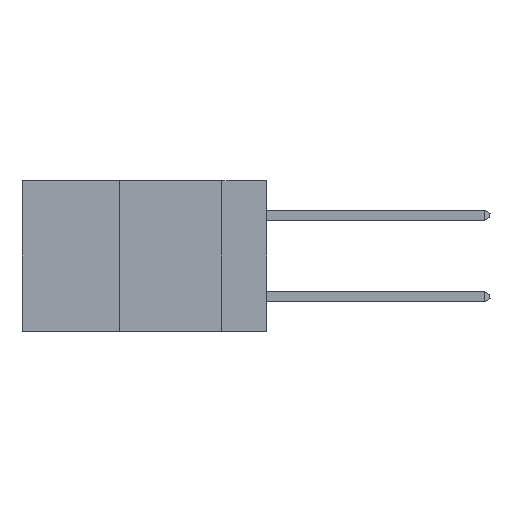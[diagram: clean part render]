
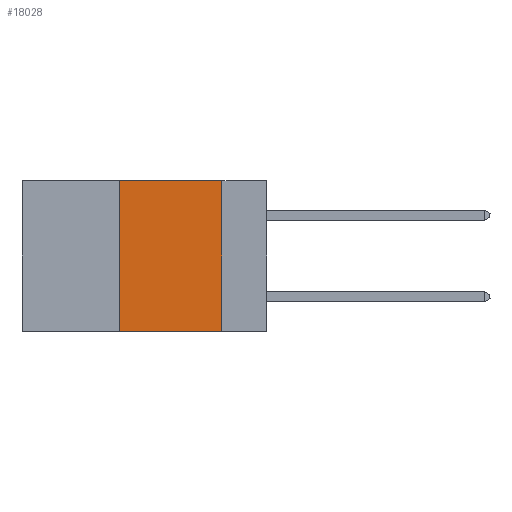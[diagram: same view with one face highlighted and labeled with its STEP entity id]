
A CAD part, left-side view. The second image highlights one B-rep face of the part: STEP entity #18028.
In plain terms, the highlighted planar face has unit normal (-1, 0, 0).
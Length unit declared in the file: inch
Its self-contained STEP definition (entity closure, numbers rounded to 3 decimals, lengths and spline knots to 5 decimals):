
#571 = ORIENTED_EDGE ( 'NONE', *, *, #4013, .T. ) ;
#1999 = CARTESIAN_POINT ( 'NONE',  ( 0., 0.6, -0.37 ) ) ;
#2124 = CARTESIAN_POINT ( 'NONE',  ( 0., 0.36, 0. ) ) ;
#2142 = EDGE_CURVE ( 'NONE', #8139, #10416, #19384, .T. ) ;
#3192 = PLANE ( 'NONE',  #8632 ) ;
#3274 = DIRECTION ( 'NONE',  ( 0., 0., -1. ) ) ;
#4013 = EDGE_CURVE ( 'NONE', #22572, #22869, #22511, .T. ) ;
#5588 = ORIENTED_EDGE ( 'NONE', *, *, #2142, .F. ) ;
#5863 = DIRECTION ( 'NONE',  ( 0., 0., -1. ) ) ;
#6243 = ORIENTED_EDGE ( 'NONE', *, *, #10483, .F. ) ;
#6394 = VECTOR ( 'NONE', #15481, 39.37008 ) ;
#6607 = EDGE_CURVE ( 'NONE', #22572, #8139, #11484, .T. ) ;
#8139 = VERTEX_POINT ( 'NONE', #15654 ) ;
#8632 = AXIS2_PLACEMENT_3D ( 'NONE', #12797, #14714, #3274 ) ;
#9438 = CARTESIAN_POINT ( 'NONE',  ( 0., 0.11, -0.37 ) ) ;
#9506 = CARTESIAN_POINT ( 'NONE',  ( 0., 0.11, 0. ) ) ;
#10416 = VERTEX_POINT ( 'NONE', #9506 ) ;
#10483 = EDGE_CURVE ( 'NONE', #10416, #22869, #19931, .T. ) ;
#11484 = LINE ( 'NONE', #2124, #6394 ) ;
#12797 = CARTESIAN_POINT ( 'NONE',  ( 0., 0.6, 0. ) ) ;
#13453 = CARTESIAN_POINT ( 'NONE',  ( 0., 0.11, 0. ) ) ;
#14714 = DIRECTION ( 'NONE',  ( 1., 0., 0. ) ) ;
#15336 = FACE_OUTER_BOUND ( 'NONE', #16802, .T. ) ;
#15481 = DIRECTION ( 'NONE',  ( 0., 0., 1. ) ) ;
#15654 = CARTESIAN_POINT ( 'NONE',  ( 0., 0.36, 0. ) ) ;
#16050 = CARTESIAN_POINT ( 'NONE',  ( 0., 0.36, -0.37 ) ) ;
#16802 = EDGE_LOOP ( 'NONE', ( #6243, #5588, #18013, #571 ) ) ;
#17532 = VECTOR ( 'NONE', #19152, 39.37008 ) ;
#17719 = CARTESIAN_POINT ( 'NONE',  ( 0., 0.6, 0. ) ) ;
#18013 = ORIENTED_EDGE ( 'NONE', *, *, #6607, .F. ) ;
#18028 = ADVANCED_FACE ( 'NONE', ( #15336 ), #3192, .F. ) ;
#19152 = DIRECTION ( 'NONE',  ( 0., -1., 0. ) ) ;
#19384 = LINE ( 'NONE', #17719, #19974 ) ;
#19590 = DIRECTION ( 'NONE',  ( 0., -1., 0. ) ) ;
#19931 = LINE ( 'NONE', #13453, #24292 ) ;
#19974 = VECTOR ( 'NONE', #19590, 39.37008 ) ;
#22511 = LINE ( 'NONE', #1999, #17532 ) ;
#22572 = VERTEX_POINT ( 'NONE', #16050 ) ;
#22869 = VERTEX_POINT ( 'NONE', #9438 ) ;
#24292 = VECTOR ( 'NONE', #5863, 39.37008 ) ;
